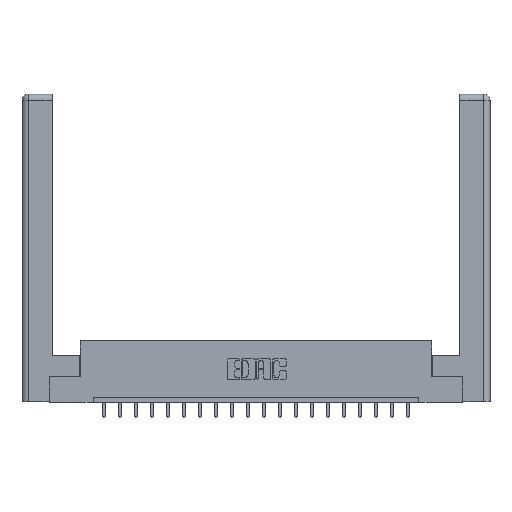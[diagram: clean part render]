
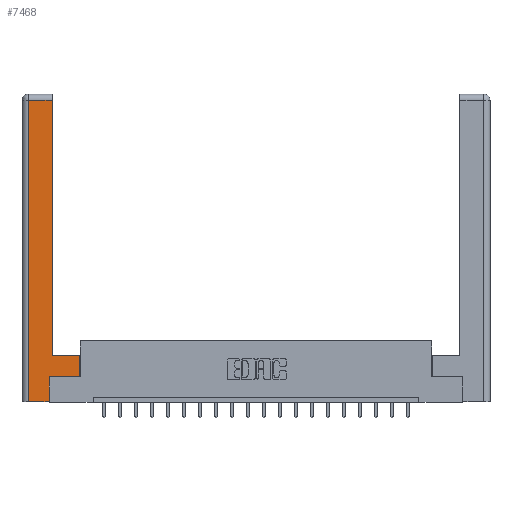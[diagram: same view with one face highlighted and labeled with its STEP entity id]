
A CAD part, top view. The second image highlights one B-rep face of the part: STEP entity #7468.
In plain terms, the highlighted planar face has unit normal (0, 0, 1).
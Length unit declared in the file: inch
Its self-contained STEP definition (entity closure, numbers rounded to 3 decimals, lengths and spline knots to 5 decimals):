
#1698 = VERTEX_POINT ( 'NONE', #17073 ) ;
#1706 = VERTEX_POINT ( 'NONE', #9031 ) ;
#1873 = CARTESIAN_POINT ( 'NONE',  ( 0.565, 0.45, 0. ) ) ;
#2171 = CARTESIAN_POINT ( 'NONE',  ( 0.295, 3., 0. ) ) ;
#2232 = EDGE_CURVE ( 'NONE', #7300, #13818, #13196, .T. ) ;
#2367 = CARTESIAN_POINT ( 'NONE',  ( 0.265, 0., 0. ) ) ;
#2393 = VERTEX_POINT ( 'NONE', #17265 ) ;
#2430 = ORIENTED_EDGE ( 'NONE', *, *, #16295, .T. ) ;
#2464 = CARTESIAN_POINT ( 'NONE',  ( 0.0615, 2.94, 0. ) ) ;
#3234 = CARTESIAN_POINT ( 'NONE',  ( 0.0615, 0., 0. ) ) ;
#3418 = EDGE_LOOP ( 'NONE', ( #13859, #12155, #13231, #2430, #3764, #18648, #6888, #7271 ) ) ;
#3764 = ORIENTED_EDGE ( 'NONE', *, *, #5439, .T. ) ;
#4465 = VECTOR ( 'NONE', #6892, 39.37008 ) ;
#5107 = VECTOR ( 'NONE', #19199, 39.37008 ) ;
#5136 = VECTOR ( 'NONE', #5215, 39.37008 ) ;
#5157 = EDGE_CURVE ( 'NONE', #10603, #7300, #15780, .T. ) ;
#5215 = DIRECTION ( 'NONE',  ( 0., 1., 0. ) ) ;
#5281 = CARTESIAN_POINT ( 'NONE',  ( 0.295, 0.45, 0. ) ) ;
#5439 = EDGE_CURVE ( 'NONE', #6116, #1698, #14268, .T. ) ;
#5519 = DIRECTION ( 'NONE',  ( 1., 0., 0. ) ) ;
#5713 = CARTESIAN_POINT ( 'NONE',  ( 0.295, 0.45, 0. ) ) ;
#5835 = VECTOR ( 'NONE', #16474, 39.37008 ) ;
#5958 = VECTOR ( 'NONE', #5519, 39.37008 ) ;
#5991 = VECTOR ( 'NONE', #14009, 39.37008 ) ;
#6116 = VERTEX_POINT ( 'NONE', #18779 ) ;
#6871 = LINE ( 'NONE', #5281, #7611 ) ;
#6888 = ORIENTED_EDGE ( 'NONE', *, *, #10451, .T. ) ;
#6892 = DIRECTION ( 'NONE',  ( 0., 1., 0. ) ) ;
#7271 = ORIENTED_EDGE ( 'NONE', *, *, #19539, .T. ) ;
#7300 = VERTEX_POINT ( 'NONE', #14904 ) ;
#7468 = ADVANCED_FACE ( 'NONE', ( #14425 ), #11935, .F. ) ;
#7611 = VECTOR ( 'NONE', #16438, 39.37008 ) ;
#8631 = LINE ( 'NONE', #1873, #4465 ) ;
#8796 = DIRECTION ( 'NONE',  ( 0., 1., 0. ) ) ;
#8863 = VECTOR ( 'NONE', #8796, 39.37008 ) ;
#9031 = CARTESIAN_POINT ( 'NONE',  ( 0.565, 0.45, 0. ) ) ;
#9236 = AXIS2_PLACEMENT_3D ( 'NONE', #13610, #18214, #12065 ) ;
#9497 = LINE ( 'NONE', #16045, #5107 ) ;
#9929 = CARTESIAN_POINT ( 'NONE',  ( 0.565, 0.245, 0. ) ) ;
#10451 = EDGE_CURVE ( 'NONE', #18901, #1706, #8631, .T. ) ;
#10603 = VERTEX_POINT ( 'NONE', #5713 ) ;
#11935 = PLANE ( 'NONE',  #9236 ) ;
#12065 = DIRECTION ( 'NONE',  ( -1., 0., 0. ) ) ;
#12155 = ORIENTED_EDGE ( 'NONE', *, *, #2232, .T. ) ;
#12408 = EDGE_CURVE ( 'NONE', #1698, #18901, #9497, .T. ) ;
#13196 = LINE ( 'NONE', #2464, #5835 ) ;
#13231 = ORIENTED_EDGE ( 'NONE', *, *, #15366, .T. ) ;
#13610 = CARTESIAN_POINT ( 'NONE',  ( 0., 0., 0. ) ) ;
#13818 = VERTEX_POINT ( 'NONE', #16528 ) ;
#13859 = ORIENTED_EDGE ( 'NONE', *, *, #5157, .T. ) ;
#14009 = DIRECTION ( 'NONE',  ( 0., -1., 0. ) ) ;
#14268 = LINE ( 'NONE', #16120, #5136 ) ;
#14316 = LINE ( 'NONE', #2367, #5958 ) ;
#14425 = FACE_OUTER_BOUND ( 'NONE', #3418, .T. ) ;
#14904 = CARTESIAN_POINT ( 'NONE',  ( 0.295, 2.94, 0. ) ) ;
#15366 = EDGE_CURVE ( 'NONE', #13818, #2393, #18531, .T. ) ;
#15780 = LINE ( 'NONE', #2171, #8863 ) ;
#16045 = CARTESIAN_POINT ( 'NONE',  ( 0.565, 0.245, 0. ) ) ;
#16120 = CARTESIAN_POINT ( 'NONE',  ( 0.265, 0.245, 0. ) ) ;
#16295 = EDGE_CURVE ( 'NONE', #2393, #6116, #14316, .T. ) ;
#16438 = DIRECTION ( 'NONE',  ( -1., 0., 0. ) ) ;
#16474 = DIRECTION ( 'NONE',  ( -1., 0., 0. ) ) ;
#16528 = CARTESIAN_POINT ( 'NONE',  ( 0.0615, 2.94, 0. ) ) ;
#17073 = CARTESIAN_POINT ( 'NONE',  ( 0.265, 0.245, 0. ) ) ;
#17265 = CARTESIAN_POINT ( 'NONE',  ( 0.0615, 0., 0. ) ) ;
#18214 = DIRECTION ( 'NONE',  ( 0., 0., -1. ) ) ;
#18531 = LINE ( 'NONE', #3234, #5991 ) ;
#18648 = ORIENTED_EDGE ( 'NONE', *, *, #12408, .T. ) ;
#18779 = CARTESIAN_POINT ( 'NONE',  ( 0.265, 0., 0. ) ) ;
#18901 = VERTEX_POINT ( 'NONE', #9929 ) ;
#19199 = DIRECTION ( 'NONE',  ( 1., 0., 0. ) ) ;
#19539 = EDGE_CURVE ( 'NONE', #1706, #10603, #6871, .T. ) ;
